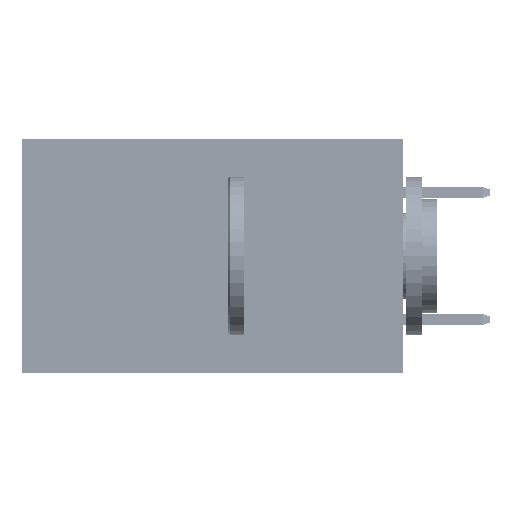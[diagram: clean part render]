
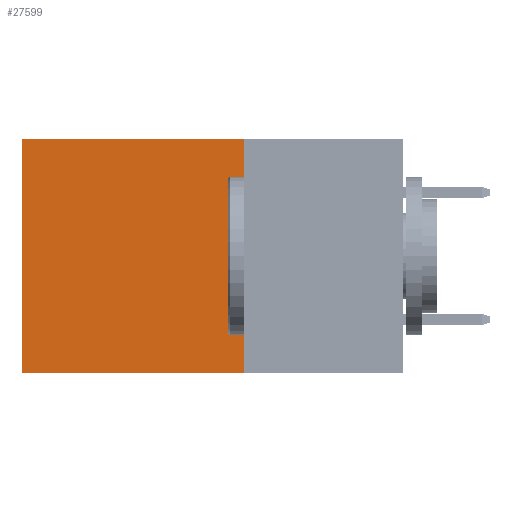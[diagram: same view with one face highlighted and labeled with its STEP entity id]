
A CAD part, left-side view. The second image highlights one B-rep face of the part: STEP entity #27599.
In plain terms, the highlighted planar face has unit normal (-1, 0, 0).
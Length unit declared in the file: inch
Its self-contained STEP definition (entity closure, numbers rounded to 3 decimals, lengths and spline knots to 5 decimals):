
#111 = EDGE_LOOP ( 'NONE', ( #34204, #34003, #45720, #17496 ) ) ;
#3246 = CARTESIAN_POINT ( 'NONE',  ( 0.2875, 0.25, -0.37 ) ) ;
#3395 = CARTESIAN_POINT ( 'NONE',  ( 0.2875, 0.6, -0.37 ) ) ;
#7584 = CARTESIAN_POINT ( 'NONE',  ( 0.2875, 0.6, 0. ) ) ;
#7761 = AXIS2_PLACEMENT_3D ( 'NONE', #40139, #47422, #19382 ) ;
#12491 = EDGE_CURVE ( 'NONE', #31005, #47158, #43788, .T. ) ;
#17496 = ORIENTED_EDGE ( 'NONE', *, *, #45130, .T. ) ;
#18509 = CARTESIAN_POINT ( 'NONE',  ( 0.2875, 0.25, -0.37 ) ) ;
#18694 = VECTOR ( 'NONE', #39674, 39.37008 ) ;
#18840 = FACE_OUTER_BOUND ( 'NONE', #111, .T. ) ;
#19382 = DIRECTION ( 'NONE',  ( 0., 0., -1. ) ) ;
#19643 = CARTESIAN_POINT ( 'NONE',  ( 0.2875, 0.25, 0. ) ) ;
#22071 = VECTOR ( 'NONE', #24514, 39.37008 ) ;
#24223 = EDGE_CURVE ( 'NONE', #47158, #31880, #44454, .T. ) ;
#24514 = DIRECTION ( 'NONE',  ( 0., 1., 0. ) ) ;
#26554 = LINE ( 'NONE', #38934, #39237 ) ;
#27599 = ADVANCED_FACE ( 'NONE', ( #18840 ), #44178, .F. ) ;
#31005 = VERTEX_POINT ( 'NONE', #19643 ) ;
#31104 = VERTEX_POINT ( 'NONE', #7584 ) ;
#31873 = LINE ( 'NONE', #43181, #18694 ) ;
#31880 = VERTEX_POINT ( 'NONE', #3395 ) ;
#32658 = VECTOR ( 'NONE', #52144, 39.37008 ) ;
#34003 = ORIENTED_EDGE ( 'NONE', *, *, #24223, .F. ) ;
#34204 = ORIENTED_EDGE ( 'NONE', *, *, #43168, .T. ) ;
#38934 = CARTESIAN_POINT ( 'NONE',  ( 0.2875, 0.6, 0. ) ) ;
#39211 = CARTESIAN_POINT ( 'NONE',  ( 0.2875, 0.25, 0. ) ) ;
#39237 = VECTOR ( 'NONE', #46182, 39.37008 ) ;
#39674 = DIRECTION ( 'NONE',  ( 0., 1., 0. ) ) ;
#40139 = CARTESIAN_POINT ( 'NONE',  ( 0.2875, 0.25, 0. ) ) ;
#43168 = EDGE_CURVE ( 'NONE', #31104, #31880, #26554, .T. ) ;
#43181 = CARTESIAN_POINT ( 'NONE',  ( 0.2875, 0.25, 0. ) ) ;
#43788 = LINE ( 'NONE', #39211, #32658 ) ;
#44178 = PLANE ( 'NONE',  #7761 ) ;
#44454 = LINE ( 'NONE', #3246, #22071 ) ;
#45130 = EDGE_CURVE ( 'NONE', #31005, #31104, #31873, .T. ) ;
#45720 = ORIENTED_EDGE ( 'NONE', *, *, #12491, .F. ) ;
#46182 = DIRECTION ( 'NONE',  ( 0., 0., -1. ) ) ;
#47158 = VERTEX_POINT ( 'NONE', #18509 ) ;
#47422 = DIRECTION ( 'NONE',  ( 1., 0., 0. ) ) ;
#52144 = DIRECTION ( 'NONE',  ( 0., 0., -1. ) ) ;
